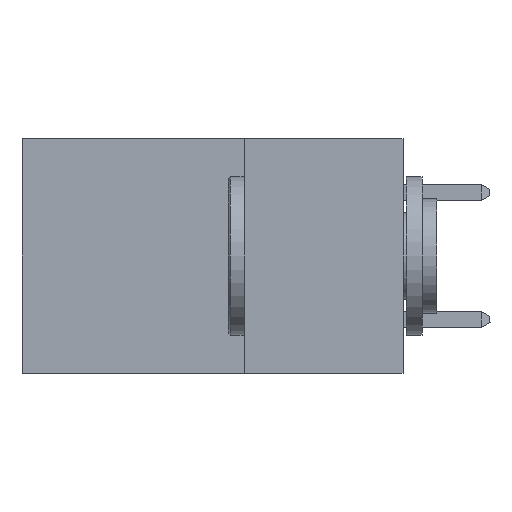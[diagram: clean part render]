
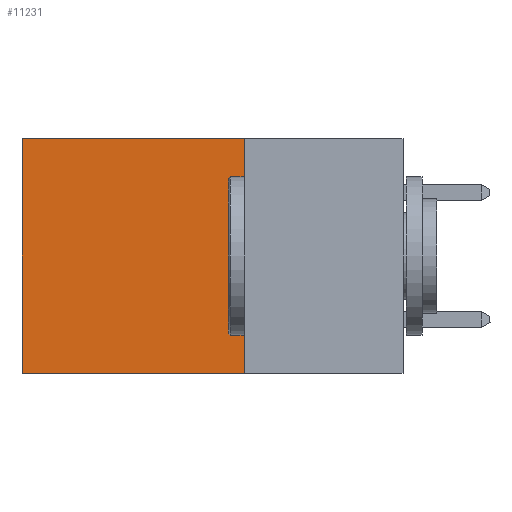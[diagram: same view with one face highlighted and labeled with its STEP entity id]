
A CAD part, left-side view. The second image highlights one B-rep face of the part: STEP entity #11231.
In plain terms, the highlighted planar face has unit normal (-1, 0, 0).
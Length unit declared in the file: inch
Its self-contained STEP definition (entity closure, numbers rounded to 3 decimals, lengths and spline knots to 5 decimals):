
#2889 = LINE ( 'NONE', #23231, #4921 ) ;
#3338 = DIRECTION ( 'NONE',  ( 0., 0., -1. ) ) ;
#4618 = ORIENTED_EDGE ( 'NONE', *, *, #33657, .T. ) ;
#4921 = VECTOR ( 'NONE', #38967, 39.37008 ) ;
#5327 = ORIENTED_EDGE ( 'NONE', *, *, #10764, .F. ) ;
#6233 = EDGE_CURVE ( 'NONE', #8512, #7325, #34345, .T. ) ;
#7325 = VERTEX_POINT ( 'NONE', #16654 ) ;
#8086 = EDGE_CURVE ( 'NONE', #8512, #34993, #21231, .T. ) ;
#8512 = VERTEX_POINT ( 'NONE', #12570 ) ;
#10300 = AXIS2_PLACEMENT_3D ( 'NONE', #16012, #32118, #12938 ) ;
#10764 = EDGE_CURVE ( 'NONE', #34993, #13490, #2889, .T. ) ;
#11231 = ADVANCED_FACE ( 'NONE', ( #19959 ), #28931, .F. ) ;
#12570 = CARTESIAN_POINT ( 'NONE',  ( 0.2875, 0.25, 0. ) ) ;
#12938 = DIRECTION ( 'NONE',  ( 0., 0., -1. ) ) ;
#13490 = VERTEX_POINT ( 'NONE', #17607 ) ;
#13934 = CARTESIAN_POINT ( 'NONE',  ( 0.2875, 0.25, 0. ) ) ;
#16012 = CARTESIAN_POINT ( 'NONE',  ( 0.2875, 0.25, 0. ) ) ;
#16318 = VECTOR ( 'NONE', #20367, 39.37008 ) ;
#16654 = CARTESIAN_POINT ( 'NONE',  ( 0.2875, 0.6, 0. ) ) ;
#17141 = CARTESIAN_POINT ( 'NONE',  ( 0.2875, 0.25, 0. ) ) ;
#17607 = CARTESIAN_POINT ( 'NONE',  ( 0.2875, 0.6, -0.37 ) ) ;
#19959 = FACE_OUTER_BOUND ( 'NONE', #28032, .T. ) ;
#20225 = VECTOR ( 'NONE', #36321, 39.37008 ) ;
#20367 = DIRECTION ( 'NONE',  ( 0., 1., 0. ) ) ;
#20832 = ORIENTED_EDGE ( 'NONE', *, *, #8086, .F. ) ;
#21231 = LINE ( 'NONE', #13934, #20225 ) ;
#23231 = CARTESIAN_POINT ( 'NONE',  ( 0.2875, 0.25, -0.37 ) ) ;
#26762 = VECTOR ( 'NONE', #3338, 39.37008 ) ;
#28032 = EDGE_LOOP ( 'NONE', ( #4618, #5327, #20832, #35477 ) ) ;
#28931 = PLANE ( 'NONE',  #10300 ) ;
#32118 = DIRECTION ( 'NONE',  ( 1., 0., 0. ) ) ;
#33657 = EDGE_CURVE ( 'NONE', #7325, #13490, #35241, .T. ) ;
#34345 = LINE ( 'NONE', #17141, #16318 ) ;
#34993 = VERTEX_POINT ( 'NONE', #35048 ) ;
#35048 = CARTESIAN_POINT ( 'NONE',  ( 0.2875, 0.25, -0.37 ) ) ;
#35241 = LINE ( 'NONE', #38500, #26762 ) ;
#35477 = ORIENTED_EDGE ( 'NONE', *, *, #6233, .T. ) ;
#36321 = DIRECTION ( 'NONE',  ( 0., 0., -1. ) ) ;
#38500 = CARTESIAN_POINT ( 'NONE',  ( 0.2875, 0.6, 0. ) ) ;
#38967 = DIRECTION ( 'NONE',  ( 0., 1., 0. ) ) ;
